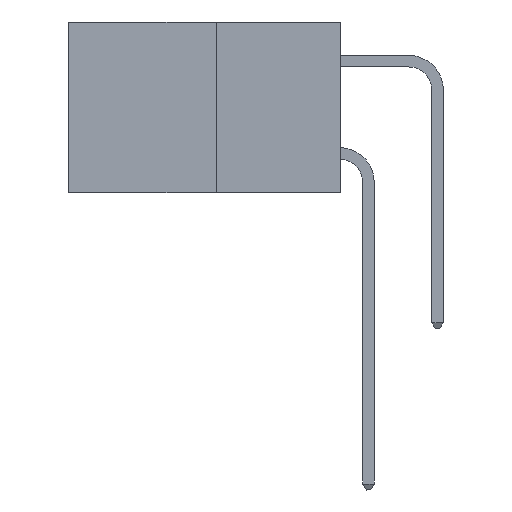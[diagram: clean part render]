
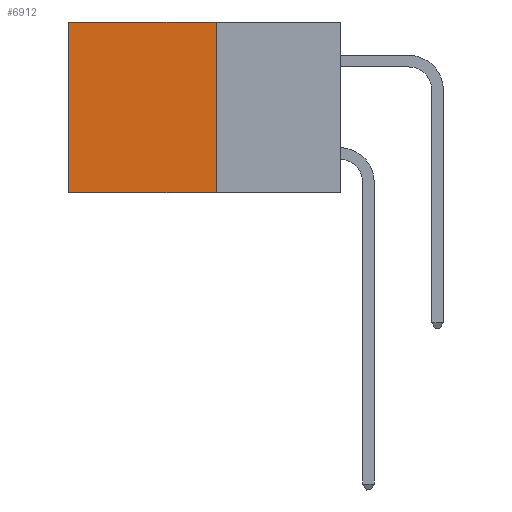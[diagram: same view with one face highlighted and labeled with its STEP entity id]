
A CAD part, left-side view. The second image highlights one B-rep face of the part: STEP entity #6912.
In plain terms, the highlighted planar face has unit normal (-1, 0, 0).
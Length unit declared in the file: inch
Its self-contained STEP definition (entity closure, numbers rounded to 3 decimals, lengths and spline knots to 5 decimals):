
#17 = VECTOR ( 'NONE', #12049, 39.37008 ) ;
#1038 = DIRECTION ( 'NONE',  ( 0., 1., 0. ) ) ;
#1057 = VERTEX_POINT ( 'NONE', #11137 ) ;
#1725 = LINE ( 'NONE', #4482, #9314 ) ;
#2254 = CARTESIAN_POINT ( 'NONE',  ( 0.277, 0.27, -0.37 ) ) ;
#2267 = EDGE_CURVE ( 'NONE', #4261, #4006, #7953, .T. ) ;
#2629 = LINE ( 'NONE', #7400, #17 ) ;
#2854 = ORIENTED_EDGE ( 'NONE', *, *, #4716, .F. ) ;
#3934 = DIRECTION ( 'NONE',  ( 0., 0., -1. ) ) ;
#3975 = DIRECTION ( 'NONE',  ( 1., 0., 0. ) ) ;
#4006 = VERTEX_POINT ( 'NONE', #4223 ) ;
#4223 = CARTESIAN_POINT ( 'NONE',  ( 0.277, 0.59, -0.37 ) ) ;
#4261 = VERTEX_POINT ( 'NONE', #5412 ) ;
#4482 = CARTESIAN_POINT ( 'NONE',  ( 0.277, 0.27, -0.37 ) ) ;
#4716 = EDGE_CURVE ( 'NONE', #8313, #4006, #1725, .T. ) ;
#5412 = CARTESIAN_POINT ( 'NONE',  ( 0.277, 0.59, 0. ) ) ;
#5430 = ORIENTED_EDGE ( 'NONE', *, *, #5589, .F. ) ;
#5494 = EDGE_LOOP ( 'NONE', ( #6342, #2854, #5430, #6040 ) ) ;
#5551 = EDGE_CURVE ( 'NONE', #1057, #4261, #2629, .T. ) ;
#5589 = EDGE_CURVE ( 'NONE', #1057, #8313, #9927, .T. ) ;
#6040 = ORIENTED_EDGE ( 'NONE', *, *, #5551, .T. ) ;
#6342 = ORIENTED_EDGE ( 'NONE', *, *, #2267, .T. ) ;
#6396 = AXIS2_PLACEMENT_3D ( 'NONE', #7770, #3975, #3934 ) ;
#6912 = ADVANCED_FACE ( 'NONE', ( #7149 ), #12175, .F. ) ;
#7149 = FACE_OUTER_BOUND ( 'NONE', #5494, .T. ) ;
#7400 = CARTESIAN_POINT ( 'NONE',  ( 0.277, 0.27, 0. ) ) ;
#7770 = CARTESIAN_POINT ( 'NONE',  ( 0.277, 0.27, -0.37 ) ) ;
#7953 = LINE ( 'NONE', #12247, #10614 ) ;
#8118 = DIRECTION ( 'NONE',  ( 0., 0., -1. ) ) ;
#8313 = VERTEX_POINT ( 'NONE', #2254 ) ;
#9314 = VECTOR ( 'NONE', #1038, 39.37008 ) ;
#9927 = LINE ( 'NONE', #12465, #12507 ) ;
#10614 = VECTOR ( 'NONE', #10772, 39.37008 ) ;
#10772 = DIRECTION ( 'NONE',  ( 0., 0., -1. ) ) ;
#11137 = CARTESIAN_POINT ( 'NONE',  ( 0.277, 0.27, 0. ) ) ;
#12049 = DIRECTION ( 'NONE',  ( 0., 1., 0. ) ) ;
#12175 = PLANE ( 'NONE',  #6396 ) ;
#12247 = CARTESIAN_POINT ( 'NONE',  ( 0.277, 0.59, -0.37 ) ) ;
#12465 = CARTESIAN_POINT ( 'NONE',  ( 0.277, 0.27, -0.37 ) ) ;
#12507 = VECTOR ( 'NONE', #8118, 39.37008 ) ;
